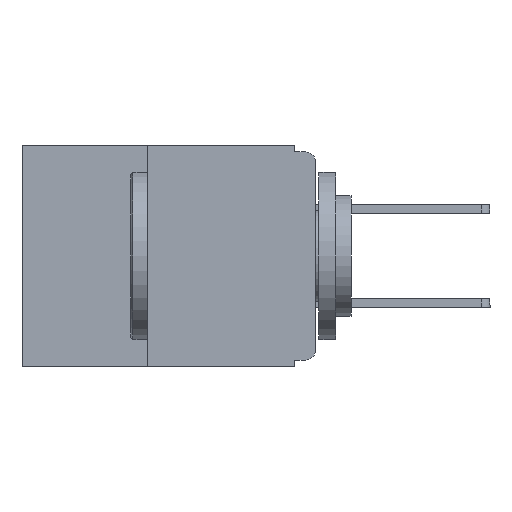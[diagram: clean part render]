
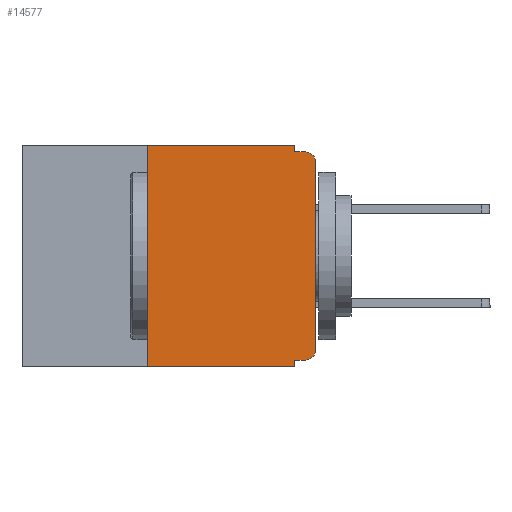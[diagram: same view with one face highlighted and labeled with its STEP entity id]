
A CAD part, left-side view. The second image highlights one B-rep face of the part: STEP entity #14577.
In plain terms, the highlighted planar face has unit normal (-1, 0, 0).
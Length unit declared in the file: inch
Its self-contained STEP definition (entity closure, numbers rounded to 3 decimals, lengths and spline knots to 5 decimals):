
#286 = VERTEX_POINT ( 'NONE', #33835 ) ;
#896 = CARTESIAN_POINT ( 'NONE',  ( 0., 0.25, -0.33 ) ) ;
#905 = DIRECTION ( 'NONE',  ( 0., 0., 1. ) ) ;
#1105 = EDGE_CURVE ( 'NONE', #3409, #12471, #30172, .T. ) ;
#1573 = CARTESIAN_POINT ( 'NONE',  ( 0., 0.015, -0.01 ) ) ;
#2444 = CARTESIAN_POINT ( 'NONE',  ( 0., 0.25, -0.33 ) ) ;
#2610 = DIRECTION ( 'NONE',  ( 0., 0., -1. ) ) ;
#3188 = EDGE_CURVE ( 'NONE', #12471, #27061, #12108, .T. ) ;
#3206 = LINE ( 'NONE', #896, #10414 ) ;
#3351 = AXIS2_PLACEMENT_3D ( 'NONE', #16499, #21817, #5705 ) ;
#3409 = VERTEX_POINT ( 'NONE', #32523 ) ;
#3903 = EDGE_CURVE ( 'NONE', #31630, #13470, #32037, .T. ) ;
#4048 = EDGE_CURVE ( 'NONE', #4197, #3409, #27036, .T. ) ;
#4197 = VERTEX_POINT ( 'NONE', #7402 ) ;
#4607 = VECTOR ( 'NONE', #18008, 39.37008 ) ;
#5015 = VERTEX_POINT ( 'NONE', #8769 ) ;
#5570 = CARTESIAN_POINT ( 'NONE',  ( 0., 0.015, -0.32 ) ) ;
#5705 = DIRECTION ( 'NONE',  ( 0., 0., -1. ) ) ;
#6365 = EDGE_CURVE ( 'NONE', #286, #12360, #30693, .T. ) ;
#7097 = CARTESIAN_POINT ( 'NONE',  ( 0., 0.031, -0.33 ) ) ;
#7256 = DIRECTION ( 'NONE',  ( 0., 0., 1. ) ) ;
#7402 = CARTESIAN_POINT ( 'NONE',  ( 0., 0.25, 0. ) ) ;
#7475 = CARTESIAN_POINT ( 'NONE',  ( 0., 0., 0. ) ) ;
#7924 = ORIENTED_EDGE ( 'NONE', *, *, #6365, .T. ) ;
#8307 = CARTESIAN_POINT ( 'NONE',  ( 0., 0., -0.01 ) ) ;
#8498 = DIRECTION ( 'NONE',  ( 0., -1., 0. ) ) ;
#8769 = CARTESIAN_POINT ( 'NONE',  ( 0., 0.031, -0.33 ) ) ;
#9675 = ORIENTED_EDGE ( 'NONE', *, *, #1105, .F. ) ;
#9753 = EDGE_CURVE ( 'NONE', #32830, #4197, #3206, .T. ) ;
#9928 = VECTOR ( 'NONE', #17362, 39.37008 ) ;
#10201 = CARTESIAN_POINT ( 'NONE',  ( 0., 0.015, -0.305 ) ) ;
#10414 = VECTOR ( 'NONE', #905, 39.37008 ) ;
#10678 = CIRCLE ( 'NONE', #32342, 0.015 ) ;
#12108 = LINE ( 'NONE', #8307, #27094 ) ;
#12360 = VERTEX_POINT ( 'NONE', #33841 ) ;
#12471 = VERTEX_POINT ( 'NONE', #23716 ) ;
#12520 = DIRECTION ( 'NONE',  ( 0., 0., -1. ) ) ;
#12655 = CARTESIAN_POINT ( 'NONE',  ( 0., 0.031, 0. ) ) ;
#12692 = LINE ( 'NONE', #7097, #4607 ) ;
#12951 = DIRECTION ( 'NONE',  ( 0., 0., -1. ) ) ;
#13068 = EDGE_CURVE ( 'NONE', #32830, #5015, #24271, .T. ) ;
#13346 = EDGE_CURVE ( 'NONE', #12360, #27061, #15192, .T. ) ;
#13470 = VERTEX_POINT ( 'NONE', #32447 ) ;
#13588 = DIRECTION ( 'NONE',  ( 0., -1., 0. ) ) ;
#13715 = CARTESIAN_POINT ( 'NONE',  ( 0., 0.437, 0. ) ) ;
#14046 = AXIS2_PLACEMENT_3D ( 'NONE', #34618, #18799, #2610 ) ;
#14421 = ORIENTED_EDGE ( 'NONE', *, *, #3903, .F. ) ;
#14577 = ADVANCED_FACE ( 'NONE', ( #18890 ), #32376, .F. ) ;
#14976 = CARTESIAN_POINT ( 'NONE',  ( 0., 0.437, -0.33 ) ) ;
#15192 = CIRCLE ( 'NONE', #14046, 0.015 ) ;
#15267 = VECTOR ( 'NONE', #12520, 39.37008 ) ;
#16436 = VECTOR ( 'NONE', #17678, 39.37008 ) ;
#16499 = CARTESIAN_POINT ( 'NONE',  ( 0., 0.437, 0. ) ) ;
#17295 = CARTESIAN_POINT ( 'NONE',  ( 0., 0., -0.32 ) ) ;
#17362 = DIRECTION ( 'NONE',  ( 0., 1., 0. ) ) ;
#17678 = DIRECTION ( 'NONE',  ( 0., -1., 0. ) ) ;
#18008 = DIRECTION ( 'NONE',  ( 0., 0., -1. ) ) ;
#18799 = DIRECTION ( 'NONE',  ( -1., 0., 0. ) ) ;
#18826 = ORIENTED_EDGE ( 'NONE', *, *, #9753, .F. ) ;
#18890 = FACE_OUTER_BOUND ( 'NONE', #28540, .T. ) ;
#19781 = ORIENTED_EDGE ( 'NONE', *, *, #3188, .F. ) ;
#21817 = DIRECTION ( 'NONE',  ( 1., 0., 0. ) ) ;
#23592 = VECTOR ( 'NONE', #7256, 39.37008 ) ;
#23716 = CARTESIAN_POINT ( 'NONE',  ( 0., 0.031, -0.01 ) ) ;
#24271 = LINE ( 'NONE', #14976, #16436 ) ;
#25361 = EDGE_CURVE ( 'NONE', #31630, #286, #10678, .T. ) ;
#26192 = VECTOR ( 'NONE', #13588, 39.37008 ) ;
#27036 = LINE ( 'NONE', #13715, #26192 ) ;
#27061 = VERTEX_POINT ( 'NONE', #1573 ) ;
#27094 = VECTOR ( 'NONE', #8498, 39.37008 ) ;
#28008 = EDGE_CURVE ( 'NONE', #13470, #5015, #12692, .T. ) ;
#28540 = EDGE_LOOP ( 'NONE', ( #7924, #30041, #19781, #9675, #32768, #18826, #33635, #32567, #14421, #31252 ) ) ;
#28851 = DIRECTION ( 'NONE',  ( -1., 0., 0. ) ) ;
#30041 = ORIENTED_EDGE ( 'NONE', *, *, #13346, .T. ) ;
#30172 = LINE ( 'NONE', #12655, #15267 ) ;
#30693 = LINE ( 'NONE', #7475, #23592 ) ;
#31252 = ORIENTED_EDGE ( 'NONE', *, *, #25361, .T. ) ;
#31630 = VERTEX_POINT ( 'NONE', #5570 ) ;
#32037 = LINE ( 'NONE', #17295, #9928 ) ;
#32342 = AXIS2_PLACEMENT_3D ( 'NONE', #10201, #28851, #12951 ) ;
#32376 = PLANE ( 'NONE',  #3351 ) ;
#32447 = CARTESIAN_POINT ( 'NONE',  ( 0., 0.031, -0.32 ) ) ;
#32523 = CARTESIAN_POINT ( 'NONE',  ( 0., 0.031, 0. ) ) ;
#32567 = ORIENTED_EDGE ( 'NONE', *, *, #28008, .F. ) ;
#32768 = ORIENTED_EDGE ( 'NONE', *, *, #4048, .F. ) ;
#32830 = VERTEX_POINT ( 'NONE', #2444 ) ;
#33635 = ORIENTED_EDGE ( 'NONE', *, *, #13068, .T. ) ;
#33835 = CARTESIAN_POINT ( 'NONE',  ( 0., 0., -0.305 ) ) ;
#33841 = CARTESIAN_POINT ( 'NONE',  ( 0., 0., -0.025 ) ) ;
#34618 = CARTESIAN_POINT ( 'NONE',  ( 0., 0.015, -0.025 ) ) ;
